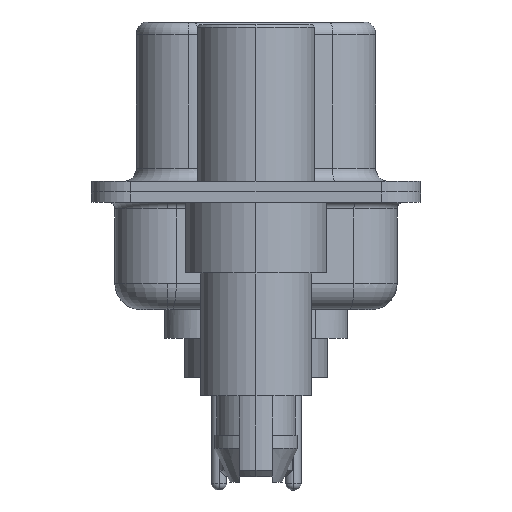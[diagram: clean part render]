
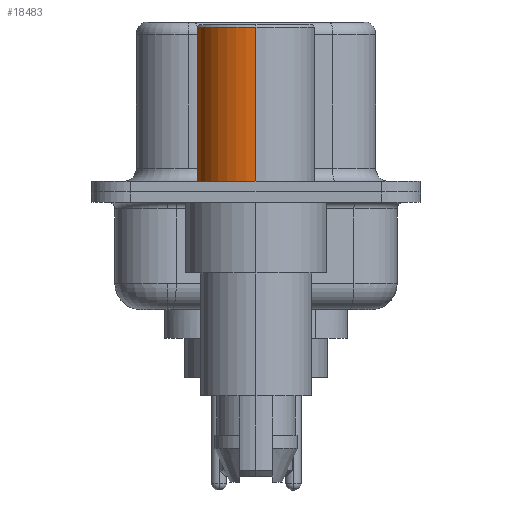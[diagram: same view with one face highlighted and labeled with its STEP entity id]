
A CAD part, left-side view. The second image highlights one B-rep face of the part: STEP entity #18483.
In plain terms, the highlighted cylindrical face has radius 2.25 mm (diameter 4.5 mm), a partial arc.
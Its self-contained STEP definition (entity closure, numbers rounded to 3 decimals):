
#411 = CARTESIAN_POINT ( 'NONE',  ( -2.25, 0., 0.4 ) ) ;
#928 = AXIS2_PLACEMENT_3D ( 'NONE', #21337, #17976, #11286 ) ;
#1122 = ORIENTED_EDGE ( 'NONE', *, *, #17703, .F. ) ;
#1654 = CIRCLE ( 'NONE', #12777, 2.25 ) ;
#1726 = VERTEX_POINT ( 'NONE', #11929 ) ;
#3633 = CARTESIAN_POINT ( 'NONE',  ( 0., 0., 6.3 ) ) ;
#3710 = EDGE_CURVE ( 'NONE', #14125, #19138, #18833, .T. ) ;
#4427 = CARTESIAN_POINT ( 'NONE',  ( 0., 0., 0.4 ) ) ;
#5245 = CIRCLE ( 'NONE', #7242, 2.25 ) ;
#5347 = DIRECTION ( 'NONE',  ( 1., 0., 0. ) ) ;
#5446 = CARTESIAN_POINT ( 'NONE',  ( 2.25, 0., 0.581 ) ) ;
#5524 = DIRECTION ( 'NONE',  ( 0., 0., 1. ) ) ;
#6139 = DIRECTION ( 'NONE',  ( 1., 0., 0. ) ) ;
#6509 = CARTESIAN_POINT ( 'NONE',  ( -2.25, 0., 0.581 ) ) ;
#7242 = AXIS2_PLACEMENT_3D ( 'NONE', #4427, #16213, #6139 ) ;
#7380 = EDGE_CURVE ( 'NONE', #9130, #14125, #5245, .T. ) ;
#8730 = CYLINDRICAL_SURFACE ( 'NONE', #928, 2.25 ) ;
#9130 = VERTEX_POINT ( 'NONE', #21025 ) ;
#9879 = VECTOR ( 'NONE', #14095, 1000. ) ;
#10817 = ORIENTED_EDGE ( 'NONE', *, *, #7380, .T. ) ;
#11083 = CARTESIAN_POINT ( 'NONE',  ( -2.25, 0., 6.3 ) ) ;
#11286 = DIRECTION ( 'NONE',  ( 1., 0., 0. ) ) ;
#11929 = CARTESIAN_POINT ( 'NONE',  ( 2.25, 0., 6.3 ) ) ;
#12777 = AXIS2_PLACEMENT_3D ( 'NONE', #3633, #15416, #5347 ) ;
#12964 = LINE ( 'NONE', #5446, #16915 ) ;
#14095 = DIRECTION ( 'NONE',  ( 0., 0., 1. ) ) ;
#14125 = VERTEX_POINT ( 'NONE', #411 ) ;
#15416 = DIRECTION ( 'NONE',  ( 0., 0., 1. ) ) ;
#15642 = EDGE_CURVE ( 'NONE', #1726, #19138, #1654, .T. ) ;
#15760 = ORIENTED_EDGE ( 'NONE', *, *, #15642, .F. ) ;
#16213 = DIRECTION ( 'NONE',  ( 0., 0., 1. ) ) ;
#16657 = ORIENTED_EDGE ( 'NONE', *, *, #3710, .T. ) ;
#16915 = VECTOR ( 'NONE', #5524, 1000. ) ;
#17669 = FACE_OUTER_BOUND ( 'NONE', #18091, .T. ) ;
#17703 = EDGE_CURVE ( 'NONE', #9130, #1726, #12964, .T. ) ;
#17976 = DIRECTION ( 'NONE',  ( 0., 0., 1. ) ) ;
#18091 = EDGE_LOOP ( 'NONE', ( #10817, #16657, #15760, #1122 ) ) ;
#18483 = ADVANCED_FACE ( 'NONE', ( #17669 ), #8730, .T. ) ;
#18833 = LINE ( 'NONE', #6509, #9879 ) ;
#19138 = VERTEX_POINT ( 'NONE', #11083 ) ;
#21025 = CARTESIAN_POINT ( 'NONE',  ( 2.25, 0., 0.4 ) ) ;
#21337 = CARTESIAN_POINT ( 'NONE',  ( 0., 0., 0.581 ) ) ;
